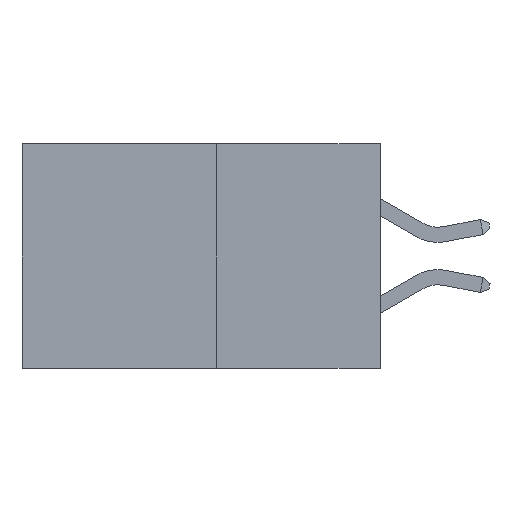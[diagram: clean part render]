
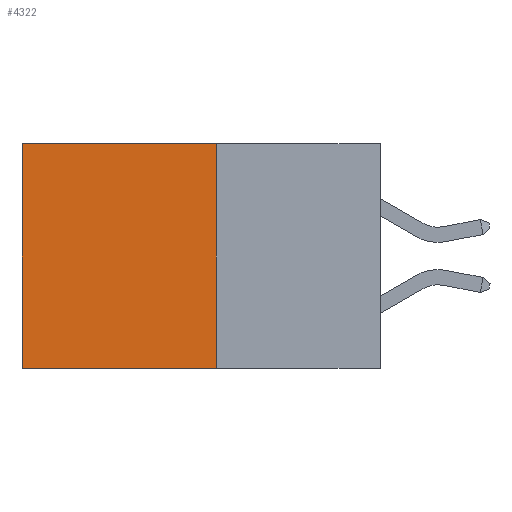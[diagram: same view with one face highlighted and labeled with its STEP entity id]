
A CAD part, left-side view. The second image highlights one B-rep face of the part: STEP entity #4322.
In plain terms, the highlighted planar face has unit normal (-1, 0, 0).
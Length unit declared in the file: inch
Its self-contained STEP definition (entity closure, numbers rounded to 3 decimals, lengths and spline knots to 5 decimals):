
#626 = VERTEX_POINT ( 'NONE', #16826 ) ;
#2233 = EDGE_CURVE ( 'NONE', #23041, #10494, #3341, .T. ) ;
#2940 = CARTESIAN_POINT ( 'NONE',  ( 0.277, 0.27, -0.37 ) ) ;
#3341 = LINE ( 'NONE', #9626, #22804 ) ;
#3848 = ORIENTED_EDGE ( 'NONE', *, *, #9688, .F. ) ;
#4103 = VERTEX_POINT ( 'NONE', #13616 ) ;
#4175 = ORIENTED_EDGE ( 'NONE', *, *, #6657, .F. ) ;
#4322 = ADVANCED_FACE ( 'NONE', ( #10076 ), #6232, .F. ) ;
#4336 = CARTESIAN_POINT ( 'NONE',  ( 0.277, 0.27, -0.37 ) ) ;
#4953 = VECTOR ( 'NONE', #14037, 39.37008 ) ;
#6232 = PLANE ( 'NONE',  #17160 ) ;
#6559 = CARTESIAN_POINT ( 'NONE',  ( 0.277, 0.27, 0. ) ) ;
#6657 = EDGE_CURVE ( 'NONE', #626, #10494, #22908, .T. ) ;
#7073 = CARTESIAN_POINT ( 'NONE',  ( 0.277, 0.59, -0.37 ) ) ;
#7837 = DIRECTION ( 'NONE',  ( 1., 0., 0. ) ) ;
#8712 = DIRECTION ( 'NONE',  ( 0., 0., -1. ) ) ;
#9151 = VECTOR ( 'NONE', #18140, 39.37008 ) ;
#9626 = CARTESIAN_POINT ( 'NONE',  ( 0.277, 0.59, -0.37 ) ) ;
#9688 = EDGE_CURVE ( 'NONE', #4103, #626, #10128, .T. ) ;
#10076 = FACE_OUTER_BOUND ( 'NONE', #17864, .T. ) ;
#10128 = LINE ( 'NONE', #4336, #4953 ) ;
#10494 = VERTEX_POINT ( 'NONE', #7073 ) ;
#12681 = VECTOR ( 'NONE', #14687, 39.37008 ) ;
#13616 = CARTESIAN_POINT ( 'NONE',  ( 0.277, 0.27, 0. ) ) ;
#13899 = CARTESIAN_POINT ( 'NONE',  ( 0.277, 0.27, -0.37 ) ) ;
#14037 = DIRECTION ( 'NONE',  ( 0., 0., -1. ) ) ;
#14687 = DIRECTION ( 'NONE',  ( 0., 1., 0. ) ) ;
#16826 = CARTESIAN_POINT ( 'NONE',  ( 0.277, 0.27, -0.37 ) ) ;
#17160 = AXIS2_PLACEMENT_3D ( 'NONE', #2940, #7837, #8712 ) ;
#17864 = EDGE_LOOP ( 'NONE', ( #19055, #4175, #3848, #19312 ) ) ;
#18140 = DIRECTION ( 'NONE',  ( 0., 1., 0. ) ) ;
#19055 = ORIENTED_EDGE ( 'NONE', *, *, #2233, .T. ) ;
#19312 = ORIENTED_EDGE ( 'NONE', *, *, #24623, .T. ) ;
#19475 = CARTESIAN_POINT ( 'NONE',  ( 0.277, 0.59, 0. ) ) ;
#22804 = VECTOR ( 'NONE', #23215, 39.37008 ) ;
#22908 = LINE ( 'NONE', #13899, #12681 ) ;
#23041 = VERTEX_POINT ( 'NONE', #19475 ) ;
#23215 = DIRECTION ( 'NONE',  ( 0., 0., -1. ) ) ;
#23922 = LINE ( 'NONE', #6559, #9151 ) ;
#24623 = EDGE_CURVE ( 'NONE', #4103, #23041, #23922, .T. ) ;
